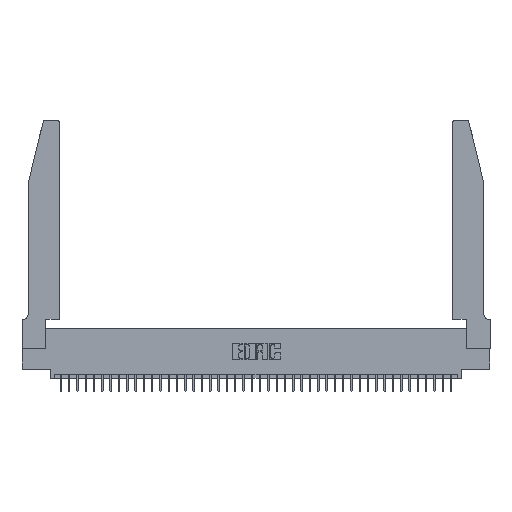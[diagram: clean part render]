
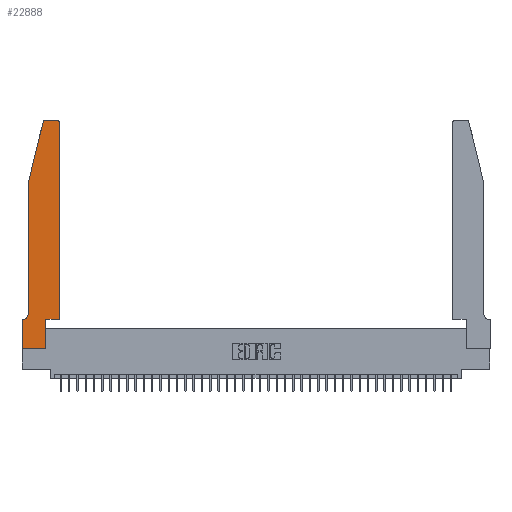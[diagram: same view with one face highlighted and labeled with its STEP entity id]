
A CAD part, top view. The second image highlights one B-rep face of the part: STEP entity #22888.
In plain terms, the highlighted planar face has unit normal (0, 0, 1).
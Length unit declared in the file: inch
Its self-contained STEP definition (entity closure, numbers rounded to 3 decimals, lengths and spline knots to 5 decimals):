
#794 = CARTESIAN_POINT ( 'NONE',  ( 0., 0., 0.37 ) ) ;
#1797 = CARTESIAN_POINT ( 'NONE',  ( 0.4505, 0.35, 0.37 ) ) ;
#1966 = LINE ( 'NONE', #1797, #35271 ) ;
#1971 = ORIENTED_EDGE ( 'NONE', *, *, #6045, .T. ) ;
#2005 = DIRECTION ( 'NONE',  ( 0., 0., 1. ) ) ;
#2080 = CIRCLE ( 'NONE', #4817, 0.07 ) ;
#2141 = VECTOR ( 'NONE', #28894, 39.37008 ) ;
#2327 = LINE ( 'NONE', #794, #16514 ) ;
#2682 = AXIS2_PLACEMENT_3D ( 'NONE', #34717, #2005, #34293 ) ;
#2796 = VERTEX_POINT ( 'NONE', #38937 ) ;
#3057 = DIRECTION ( 'NONE',  ( -1., 0., 0. ) ) ;
#3358 = LINE ( 'NONE', #29034, #31151 ) ;
#3723 = CARTESIAN_POINT ( 'NONE',  ( 0.4505, 2.72, 0.37 ) ) ;
#4355 = VERTEX_POINT ( 'NONE', #29478 ) ;
#4814 = VECTOR ( 'NONE', #30431, 39.37008 ) ;
#4817 = AXIS2_PLACEMENT_3D ( 'NONE', #38316, #18735, #3057 ) ;
#5015 = EDGE_CURVE ( 'NONE', #34833, #18889, #1966, .T. ) ;
#5830 = CARTESIAN_POINT ( 'NONE',  ( 0.0755, 0.35, 0.37 ) ) ;
#6045 = EDGE_CURVE ( 'NONE', #4355, #40114, #19603, .T. ) ;
#6690 = LINE ( 'NONE', #32122, #2141 ) ;
#7193 = DIRECTION ( 'NONE',  ( 1., 0., 0. ) ) ;
#7582 = DIRECTION ( 'NONE',  ( 1., 0., 0. ) ) ;
#9223 = FACE_OUTER_BOUND ( 'NONE', #34645, .T. ) ;
#9533 = ORIENTED_EDGE ( 'NONE', *, *, #5015, .T. ) ;
#9672 = CIRCLE ( 'NONE', #2682, 0.03 ) ;
#9883 = ORIENTED_EDGE ( 'NONE', *, *, #39950, .T. ) ;
#10453 = VECTOR ( 'NONE', #22912, 39.37008 ) ;
#10944 = CARTESIAN_POINT ( 'NONE',  ( 0.4205, 2.75, 0.37 ) ) ;
#11661 = CARTESIAN_POINT ( 'NONE',  ( 0.4505, 0.35, 0.37 ) ) ;
#11986 = VERTEX_POINT ( 'NONE', #22528 ) ;
#12050 = CARTESIAN_POINT ( 'NONE',  ( 0.2865, 0.35, 0.37 ) ) ;
#12367 = VECTOR ( 'NONE', #18965, 39.37008 ) ;
#12548 = CARTESIAN_POINT ( 'NONE',  ( 0.284, 2.75, 0.37 ) ) ;
#13130 = CARTESIAN_POINT ( 'NONE',  ( 0.0755, 2., 0.37 ) ) ;
#14874 = VERTEX_POINT ( 'NONE', #3723 ) ;
#14984 = DIRECTION ( 'NONE',  ( 1., 0., 0. ) ) ;
#15848 = EDGE_CURVE ( 'NONE', #11986, #20725, #2327, .T. ) ;
#16278 = EDGE_CURVE ( 'NONE', #18680, #4355, #20959, .T. ) ;
#16514 = VECTOR ( 'NONE', #7582, 39.37008 ) ;
#16747 = CARTESIAN_POINT ( 'NONE',  ( 0.0755, 0.42, 0.37 ) ) ;
#18680 = VERTEX_POINT ( 'NONE', #31661 ) ;
#18735 = DIRECTION ( 'NONE',  ( 0., 0., -1. ) ) ;
#18817 = CARTESIAN_POINT ( 'NONE',  ( 0., 0.35, 0.37 ) ) ;
#18889 = VERTEX_POINT ( 'NONE', #35673 ) ;
#18965 = DIRECTION ( 'NONE',  ( 0., 1., 0. ) ) ;
#19603 = LINE ( 'NONE', #40585, #25670 ) ;
#19840 = EDGE_CURVE ( 'NONE', #18889, #14874, #32100, .T. ) ;
#20725 = VERTEX_POINT ( 'NONE', #28126 ) ;
#20791 = EDGE_CURVE ( 'NONE', #20725, #34833, #35492, .T. ) ;
#20959 = LINE ( 'NONE', #13130, #41724 ) ;
#21256 = DIRECTION ( 'NONE',  ( 0., -1., 0. ) ) ;
#22201 = PLANE ( 'NONE',  #35426 ) ;
#22528 = CARTESIAN_POINT ( 'NONE',  ( 0., 0., 0.37 ) ) ;
#22888 = ADVANCED_FACE ( 'NONE', ( #9223 ), #22201, .T. ) ;
#22912 = DIRECTION ( 'NONE',  ( -1., 0., 0. ) ) ;
#23682 = CARTESIAN_POINT ( 'NONE',  ( 0., 0.35, 0.37 ) ) ;
#25670 = VECTOR ( 'NONE', #21256, 39.37008 ) ;
#26416 = ORIENTED_EDGE ( 'NONE', *, *, #15848, .T. ) ;
#27133 = ORIENTED_EDGE ( 'NONE', *, *, #34672, .T. ) ;
#28126 = CARTESIAN_POINT ( 'NONE',  ( 0.2865, 0., 0.37 ) ) ;
#28786 = EDGE_CURVE ( 'NONE', #30340, #34216, #3358, .T. ) ;
#28894 = DIRECTION ( 'NONE',  ( 0., -1., 0. ) ) ;
#29034 = CARTESIAN_POINT ( 'NONE',  ( 0.2605, 2.75, 0.37 ) ) ;
#29175 = DIRECTION ( 'NONE',  ( -1., 0., 0. ) ) ;
#29478 = CARTESIAN_POINT ( 'NONE',  ( 0.0755, 2., 0.37 ) ) ;
#29481 = ORIENTED_EDGE ( 'NONE', *, *, #20791, .T. ) ;
#30340 = VERTEX_POINT ( 'NONE', #10944 ) ;
#30431 = DIRECTION ( 'NONE',  ( 0., 1., 0. ) ) ;
#30626 = ORIENTED_EDGE ( 'NONE', *, *, #28786, .T. ) ;
#31151 = VECTOR ( 'NONE', #29175, 39.37008 ) ;
#31517 = CARTESIAN_POINT ( 'NONE',  ( 0.2865, 0.35, 0.37 ) ) ;
#31661 = CARTESIAN_POINT ( 'NONE',  ( 0.25487, 2.72718, 0.37 ) ) ;
#32100 = LINE ( 'NONE', #11661, #4814 ) ;
#32122 = CARTESIAN_POINT ( 'NONE',  ( 0., 0., 0.37 ) ) ;
#32182 = ORIENTED_EDGE ( 'NONE', *, *, #16278, .T. ) ;
#32471 = ORIENTED_EDGE ( 'NONE', *, *, #34974, .T. ) ;
#32722 = ORIENTED_EDGE ( 'NONE', *, *, #19840, .T. ) ;
#32883 = CARTESIAN_POINT ( 'NONE',  ( 0.284, 2.72, 0.37 ) ) ;
#33360 = VERTEX_POINT ( 'NONE', #23682 ) ;
#33731 = AXIS2_PLACEMENT_3D ( 'NONE', #32883, #38821, #7193 ) ;
#34112 = EDGE_CURVE ( 'NONE', #40114, #2796, #2080, .T. ) ;
#34216 = VERTEX_POINT ( 'NONE', #12548 ) ;
#34293 = DIRECTION ( 'NONE',  ( 1., 0., 0. ) ) ;
#34546 = DIRECTION ( 'NONE',  ( 0., 0., 1. ) ) ;
#34645 = EDGE_LOOP ( 'NONE', ( #30626, #32471, #32182, #1971, #36642, #39166, #9883, #26416, #29481, #9533, #32722, #27133 ) ) ;
#34672 = EDGE_CURVE ( 'NONE', #14874, #30340, #9672, .T. ) ;
#34705 = DIRECTION ( 'NONE',  ( 1., 0., 0. ) ) ;
#34717 = CARTESIAN_POINT ( 'NONE',  ( 0.4205, 2.72, 0.37 ) ) ;
#34833 = VERTEX_POINT ( 'NONE', #12050 ) ;
#34974 = EDGE_CURVE ( 'NONE', #34216, #18680, #41449, .T. ) ;
#35271 = VECTOR ( 'NONE', #14984, 39.37008 ) ;
#35426 = AXIS2_PLACEMENT_3D ( 'NONE', #18817, #34546, #34705 ) ;
#35492 = LINE ( 'NONE', #31517, #12367 ) ;
#35673 = CARTESIAN_POINT ( 'NONE',  ( 0.4505, 0.35, 0.37 ) ) ;
#36281 = DIRECTION ( 'NONE',  ( -0.239, -0.971, 0. ) ) ;
#36642 = ORIENTED_EDGE ( 'NONE', *, *, #34112, .T. ) ;
#36731 = EDGE_CURVE ( 'NONE', #2796, #33360, #37150, .T. ) ;
#37150 = LINE ( 'NONE', #5830, #10453 ) ;
#38316 = CARTESIAN_POINT ( 'NONE',  ( 0.0055, 0.42, 0.37 ) ) ;
#38821 = DIRECTION ( 'NONE',  ( 0., 0., 1. ) ) ;
#38937 = CARTESIAN_POINT ( 'NONE',  ( 0.0055, 0.35, 0.37 ) ) ;
#39166 = ORIENTED_EDGE ( 'NONE', *, *, #36731, .T. ) ;
#39950 = EDGE_CURVE ( 'NONE', #33360, #11986, #6690, .T. ) ;
#40114 = VERTEX_POINT ( 'NONE', #16747 ) ;
#40585 = CARTESIAN_POINT ( 'NONE',  ( 0.0755, 2., 0.37 ) ) ;
#41449 = CIRCLE ( 'NONE', #33731, 0.03 ) ;
#41724 = VECTOR ( 'NONE', #36281, 39.37008 ) ;
